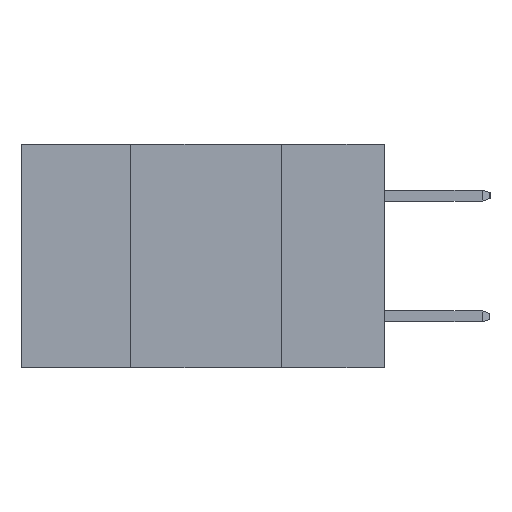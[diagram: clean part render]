
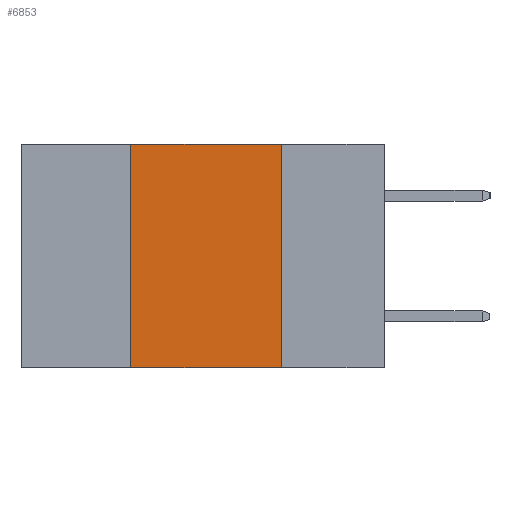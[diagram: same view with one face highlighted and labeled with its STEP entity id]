
A CAD part, left-side view. The second image highlights one B-rep face of the part: STEP entity #6853.
In plain terms, the highlighted planar face has unit normal (-1, 0, 0).
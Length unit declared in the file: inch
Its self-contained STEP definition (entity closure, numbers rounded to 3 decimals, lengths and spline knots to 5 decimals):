
#183 = AXIS2_PLACEMENT_3D ( 'NONE', #5454, #20200, #6945 ) ;
#533 = EDGE_CURVE ( 'NONE', #5808, #8512, #17976, .T. ) ;
#1707 = VERTEX_POINT ( 'NONE', #11199 ) ;
#2025 = DIRECTION ( 'NONE',  ( 0., -1., 0. ) ) ;
#3299 = ORIENTED_EDGE ( 'NONE', *, *, #19136, .F. ) ;
#4526 = DIRECTION ( 'NONE',  ( 0., 0., -1. ) ) ;
#4764 = ORIENTED_EDGE ( 'NONE', *, *, #11497, .T. ) ;
#5454 = CARTESIAN_POINT ( 'NONE',  ( 0., 0.6, 0. ) ) ;
#5559 = EDGE_CURVE ( 'NONE', #8512, #1707, #6164, .T. ) ;
#5808 = VERTEX_POINT ( 'NONE', #8245 ) ;
#6164 = LINE ( 'NONE', #17753, #8295 ) ;
#6853 = ADVANCED_FACE ( 'NONE', ( #18997 ), #15239, .F. ) ;
#6945 = DIRECTION ( 'NONE',  ( 0., 0., -1. ) ) ;
#7077 = CARTESIAN_POINT ( 'NONE',  ( 0., 0.17, -0.37 ) ) ;
#7809 = DIRECTION ( 'NONE',  ( 0., 0., 1. ) ) ;
#8089 = VECTOR ( 'NONE', #7809, 39.37008 ) ;
#8245 = CARTESIAN_POINT ( 'NONE',  ( 0., 0.42, -0.37 ) ) ;
#8295 = VECTOR ( 'NONE', #19270, 39.37008 ) ;
#8512 = VERTEX_POINT ( 'NONE', #18690 ) ;
#8715 = VERTEX_POINT ( 'NONE', #7077 ) ;
#9462 = VECTOR ( 'NONE', #4526, 39.37008 ) ;
#10527 = LINE ( 'NONE', #18589, #14877 ) ;
#11199 = CARTESIAN_POINT ( 'NONE',  ( 0., 0.17, 0. ) ) ;
#11497 = EDGE_CURVE ( 'NONE', #5808, #8715, #10527, .T. ) ;
#12586 = ORIENTED_EDGE ( 'NONE', *, *, #533, .F. ) ;
#14877 = VECTOR ( 'NONE', #2025, 39.37008 ) ;
#15239 = PLANE ( 'NONE',  #183 ) ;
#15976 = LINE ( 'NONE', #19617, #9462 ) ;
#16198 = CARTESIAN_POINT ( 'NONE',  ( 0., 0.42, -0.37 ) ) ;
#17107 = ORIENTED_EDGE ( 'NONE', *, *, #5559, .F. ) ;
#17753 = CARTESIAN_POINT ( 'NONE',  ( 0., 0.6, 0. ) ) ;
#17976 = LINE ( 'NONE', #16198, #8089 ) ;
#18589 = CARTESIAN_POINT ( 'NONE',  ( 0., 0.6, -0.37 ) ) ;
#18690 = CARTESIAN_POINT ( 'NONE',  ( 0., 0.42, 0. ) ) ;
#18997 = FACE_OUTER_BOUND ( 'NONE', #19261, .T. ) ;
#19136 = EDGE_CURVE ( 'NONE', #1707, #8715, #15976, .T. ) ;
#19261 = EDGE_LOOP ( 'NONE', ( #3299, #17107, #12586, #4764 ) ) ;
#19270 = DIRECTION ( 'NONE',  ( 0., -1., 0. ) ) ;
#19617 = CARTESIAN_POINT ( 'NONE',  ( 0., 0.17, -0.37 ) ) ;
#20200 = DIRECTION ( 'NONE',  ( 1., 0., 0. ) ) ;
